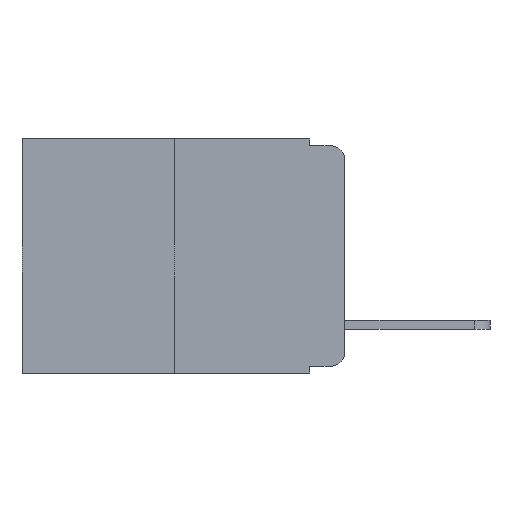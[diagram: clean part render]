
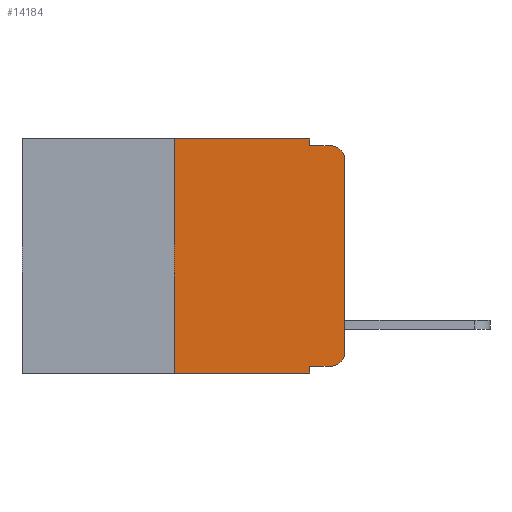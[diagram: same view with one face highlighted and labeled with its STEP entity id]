
A CAD part, left-side view. The second image highlights one B-rep face of the part: STEP entity #14184.
In plain terms, the highlighted planar face has unit normal (-1, 0, 0).
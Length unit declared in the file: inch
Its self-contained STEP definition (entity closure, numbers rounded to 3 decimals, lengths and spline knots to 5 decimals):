
#356 = ORIENTED_EDGE ( 'NONE', *, *, #15236, .T. ) ;
#367 = VECTOR ( 'NONE', #6335, 39.37008 ) ;
#418 = EDGE_CURVE ( 'NONE', #5734, #12045, #3459, .T. ) ;
#1480 = DIRECTION ( 'NONE',  ( 0., 0., -1. ) ) ;
#1502 = DIRECTION ( 'NONE',  ( -1., 0., 0. ) ) ;
#1506 = CARTESIAN_POINT ( 'NONE',  ( 0., 0.02, -0.03 ) ) ;
#1841 = ORIENTED_EDGE ( 'NONE', *, *, #5370, .T. ) ;
#2407 = EDGE_CURVE ( 'NONE', #18156, #17368, #5291, .T. ) ;
#2715 = EDGE_LOOP ( 'NONE', ( #1841, #7430, #6232, #11854, #3386, #6793, #17382, #13414, #10019, #356 ) ) ;
#2866 = VECTOR ( 'NONE', #3484, 39.37008 ) ;
#3104 = VECTOR ( 'NONE', #9580, 39.37008 ) ;
#3379 = CARTESIAN_POINT ( 'NONE',  ( 0., 0.051, 0. ) ) ;
#3386 = ORIENTED_EDGE ( 'NONE', *, *, #15398, .F. ) ;
#3459 = LINE ( 'NONE', #3379, #2866 ) ;
#3484 = DIRECTION ( 'NONE',  ( 0., 0., -1. ) ) ;
#3542 = LINE ( 'NONE', #5287, #11656 ) ;
#3625 = VECTOR ( 'NONE', #19639, 39.37008 ) ;
#3775 = EDGE_CURVE ( 'NONE', #8155, #10979, #16891, .T. ) ;
#4364 = LINE ( 'NONE', #18084, #8247 ) ;
#4498 = CARTESIAN_POINT ( 'NONE',  ( 0., 0.051, -0.343 ) ) ;
#5287 = CARTESIAN_POINT ( 'NONE',  ( 0., 0.051, -0.333 ) ) ;
#5291 = LINE ( 'NONE', #13468, #19865 ) ;
#5370 = EDGE_CURVE ( 'NONE', #11500, #8155, #19027, .T. ) ;
#5471 = PLANE ( 'NONE',  #15245 ) ;
#5734 = VERTEX_POINT ( 'NONE', #11750 ) ;
#5735 = VERTEX_POINT ( 'NONE', #14741 ) ;
#6179 = CARTESIAN_POINT ( 'NONE',  ( 0., 0.02, -0.01 ) ) ;
#6232 = ORIENTED_EDGE ( 'NONE', *, *, #19728, .F. ) ;
#6335 = DIRECTION ( 'NONE',  ( 0., -1., 0. ) ) ;
#6793 = ORIENTED_EDGE ( 'NONE', *, *, #2407, .F. ) ;
#6961 = DIRECTION ( 'NONE',  ( 0., -1., 0. ) ) ;
#7430 = ORIENTED_EDGE ( 'NONE', *, *, #3775, .T. ) ;
#7914 = CARTESIAN_POINT ( 'NONE',  ( 0., 0.473, -0.343 ) ) ;
#8142 = AXIS2_PLACEMENT_3D ( 'NONE', #1506, #1502, #1480 ) ;
#8155 = VERTEX_POINT ( 'NONE', #8710 ) ;
#8247 = VECTOR ( 'NONE', #19473, 39.37008 ) ;
#8598 = LINE ( 'NONE', #13947, #3625 ) ;
#8710 = CARTESIAN_POINT ( 'NONE',  ( 0., 0., -0.03 ) ) ;
#8749 = DIRECTION ( 'NONE',  ( 0., 0., -1. ) ) ;
#9137 = DIRECTION ( 'NONE',  ( -1., 0., 0. ) ) ;
#9193 = EDGE_CURVE ( 'NONE', #14904, #17928, #20169, .T. ) ;
#9453 = LINE ( 'NONE', #7914, #367 ) ;
#9580 = DIRECTION ( 'NONE',  ( 0., 0., 1. ) ) ;
#10019 = ORIENTED_EDGE ( 'NONE', *, *, #11245, .T. ) ;
#10957 = CARTESIAN_POINT ( 'NONE',  ( 0., 0.051, 0. ) ) ;
#10979 = VERTEX_POINT ( 'NONE', #6179 ) ;
#11245 = EDGE_CURVE ( 'NONE', #14904, #5735, #3542, .T. ) ;
#11500 = VERTEX_POINT ( 'NONE', #15719 ) ;
#11656 = VECTOR ( 'NONE', #6961, 39.37008 ) ;
#11750 = CARTESIAN_POINT ( 'NONE',  ( 0., 0.051, 0. ) ) ;
#11854 = ORIENTED_EDGE ( 'NONE', *, *, #418, .F. ) ;
#12045 = VERTEX_POINT ( 'NONE', #19779 ) ;
#12866 = CARTESIAN_POINT ( 'NONE',  ( 0., 0.051, -0.333 ) ) ;
#13414 = ORIENTED_EDGE ( 'NONE', *, *, #9193, .F. ) ;
#13468 = CARTESIAN_POINT ( 'NONE',  ( 0., 0.25, 0. ) ) ;
#13616 = DIRECTION ( 'NONE',  ( 0., 0., 1. ) ) ;
#13773 = AXIS2_PLACEMENT_3D ( 'NONE', #18013, #9137, #19400 ) ;
#13947 = CARTESIAN_POINT ( 'NONE',  ( 0., 0.473, 0. ) ) ;
#14184 = ADVANCED_FACE ( 'NONE', ( #18154 ), #5471, .F. ) ;
#14417 = CARTESIAN_POINT ( 'NONE',  ( 0., 0.25, -0.343 ) ) ;
#14741 = CARTESIAN_POINT ( 'NONE',  ( 0., 0.02, -0.333 ) ) ;
#14904 = VERTEX_POINT ( 'NONE', #12866 ) ;
#15236 = EDGE_CURVE ( 'NONE', #5735, #11500, #18325, .T. ) ;
#15245 = AXIS2_PLACEMENT_3D ( 'NONE', #16203, #17641, #8749 ) ;
#15398 = EDGE_CURVE ( 'NONE', #17368, #5734, #8598, .T. ) ;
#15719 = CARTESIAN_POINT ( 'NONE',  ( 0., 0., -0.313 ) ) ;
#15979 = VECTOR ( 'NONE', #18302, 39.37008 ) ;
#16203 = CARTESIAN_POINT ( 'NONE',  ( 0., 0.473, 0. ) ) ;
#16891 = CIRCLE ( 'NONE', #8142, 0.02 ) ;
#17102 = CARTESIAN_POINT ( 'NONE',  ( 0., 0., 0. ) ) ;
#17368 = VERTEX_POINT ( 'NONE', #18215 ) ;
#17382 = ORIENTED_EDGE ( 'NONE', *, *, #19880, .T. ) ;
#17641 = DIRECTION ( 'NONE',  ( 1., 0., 0. ) ) ;
#17928 = VERTEX_POINT ( 'NONE', #4498 ) ;
#18013 = CARTESIAN_POINT ( 'NONE',  ( 0., 0.02, -0.313 ) ) ;
#18084 = CARTESIAN_POINT ( 'NONE',  ( 0., 0.051, -0.01 ) ) ;
#18154 = FACE_OUTER_BOUND ( 'NONE', #2715, .T. ) ;
#18156 = VERTEX_POINT ( 'NONE', #14417 ) ;
#18215 = CARTESIAN_POINT ( 'NONE',  ( 0., 0.25, 0. ) ) ;
#18302 = DIRECTION ( 'NONE',  ( 0., 0., -1. ) ) ;
#18325 = CIRCLE ( 'NONE', #13773, 0.02 ) ;
#19027 = LINE ( 'NONE', #17102, #3104 ) ;
#19400 = DIRECTION ( 'NONE',  ( 0., 0., -1. ) ) ;
#19473 = DIRECTION ( 'NONE',  ( 0., -1., 0. ) ) ;
#19639 = DIRECTION ( 'NONE',  ( 0., -1., 0. ) ) ;
#19728 = EDGE_CURVE ( 'NONE', #12045, #10979, #4364, .T. ) ;
#19779 = CARTESIAN_POINT ( 'NONE',  ( 0., 0.051, -0.01 ) ) ;
#19865 = VECTOR ( 'NONE', #13616, 39.37008 ) ;
#19880 = EDGE_CURVE ( 'NONE', #18156, #17928, #9453, .T. ) ;
#20169 = LINE ( 'NONE', #10957, #15979 ) ;
